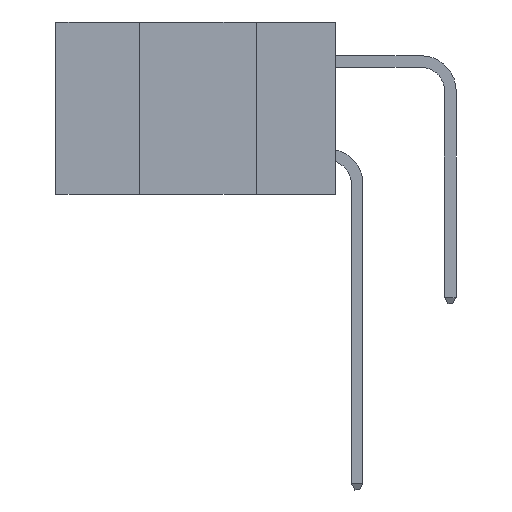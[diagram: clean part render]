
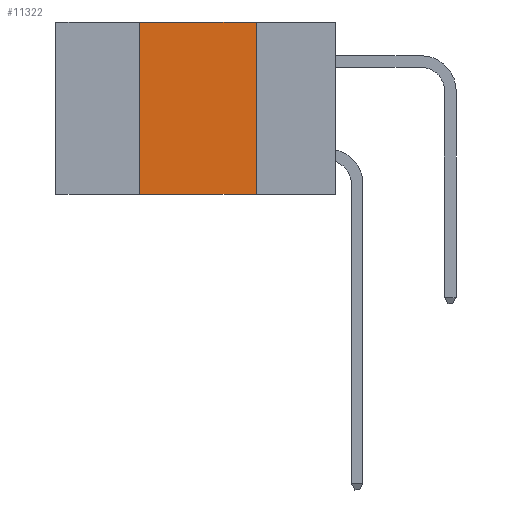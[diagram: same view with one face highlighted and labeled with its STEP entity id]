
A CAD part, left-side view. The second image highlights one B-rep face of the part: STEP entity #11322.
In plain terms, the highlighted planar face has unit normal (-1, 0, 0).
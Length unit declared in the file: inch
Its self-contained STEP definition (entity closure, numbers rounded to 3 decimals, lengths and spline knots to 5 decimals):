
#1046 = ORIENTED_EDGE ( 'NONE', *, *, #6875, .F. ) ;
#1253 = DIRECTION ( 'NONE',  ( 0., -1., 0. ) ) ;
#1304 = CARTESIAN_POINT ( 'NONE',  ( 0., 0.42, -0.37 ) ) ;
#2785 = VECTOR ( 'NONE', #1253, 39.37008 ) ;
#3314 = EDGE_CURVE ( 'NONE', #10804, #15628, #5049, .T. ) ;
#3758 = DIRECTION ( 'NONE',  ( 0., 0., -1. ) ) ;
#4644 = ORIENTED_EDGE ( 'NONE', *, *, #8850, .F. ) ;
#5028 = DIRECTION ( 'NONE',  ( 0., 0., 1. ) ) ;
#5049 = LINE ( 'NONE', #9919, #14865 ) ;
#5158 = DIRECTION ( 'NONE',  ( 1., 0., 0. ) ) ;
#5212 = CARTESIAN_POINT ( 'NONE',  ( 0., 0.6, 0. ) ) ;
#6476 = CARTESIAN_POINT ( 'NONE',  ( 0., 0.42, 0. ) ) ;
#6582 = LINE ( 'NONE', #13906, #2785 ) ;
#6651 = ORIENTED_EDGE ( 'NONE', *, *, #3314, .F. ) ;
#6875 = EDGE_CURVE ( 'NONE', #15628, #7679, #16036, .T. ) ;
#7679 = VERTEX_POINT ( 'NONE', #8760 ) ;
#8054 = EDGE_LOOP ( 'NONE', ( #1046, #6651, #4644, #9995 ) ) ;
#8204 = EDGE_CURVE ( 'NONE', #16392, #7679, #6582, .T. ) ;
#8692 = FACE_OUTER_BOUND ( 'NONE', #8054, .T. ) ;
#8760 = CARTESIAN_POINT ( 'NONE',  ( 0., 0.17, -0.37 ) ) ;
#8778 = DIRECTION ( 'NONE',  ( 0., 0., -1. ) ) ;
#8850 = EDGE_CURVE ( 'NONE', #16392, #10804, #14986, .T. ) ;
#9421 = VECTOR ( 'NONE', #8778, 39.37008 ) ;
#9919 = CARTESIAN_POINT ( 'NONE',  ( 0., 0.6, 0. ) ) ;
#9995 = ORIENTED_EDGE ( 'NONE', *, *, #8204, .T. ) ;
#10804 = VERTEX_POINT ( 'NONE', #11624 ) ;
#11322 = ADVANCED_FACE ( 'NONE', ( #8692 ), #12774, .F. ) ;
#11624 = CARTESIAN_POINT ( 'NONE',  ( 0., 0.42, 0. ) ) ;
#12774 = PLANE ( 'NONE',  #14903 ) ;
#12776 = VECTOR ( 'NONE', #5028, 39.37008 ) ;
#13207 = CARTESIAN_POINT ( 'NONE',  ( 0., 0.17, 0. ) ) ;
#13906 = CARTESIAN_POINT ( 'NONE',  ( 0., 0.6, -0.37 ) ) ;
#14865 = VECTOR ( 'NONE', #15176, 39.37008 ) ;
#14903 = AXIS2_PLACEMENT_3D ( 'NONE', #5212, #5158, #3758 ) ;
#14986 = LINE ( 'NONE', #6476, #12776 ) ;
#15176 = DIRECTION ( 'NONE',  ( 0., -1., 0. ) ) ;
#15628 = VERTEX_POINT ( 'NONE', #13207 ) ;
#16036 = LINE ( 'NONE', #16441, #9421 ) ;
#16392 = VERTEX_POINT ( 'NONE', #1304 ) ;
#16441 = CARTESIAN_POINT ( 'NONE',  ( 0., 0.17, 0. ) ) ;
